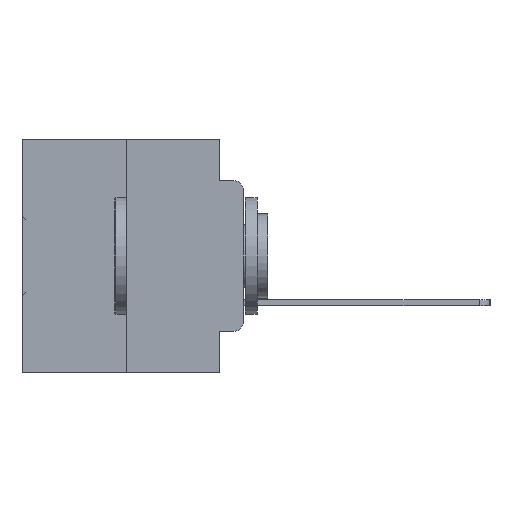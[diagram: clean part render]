
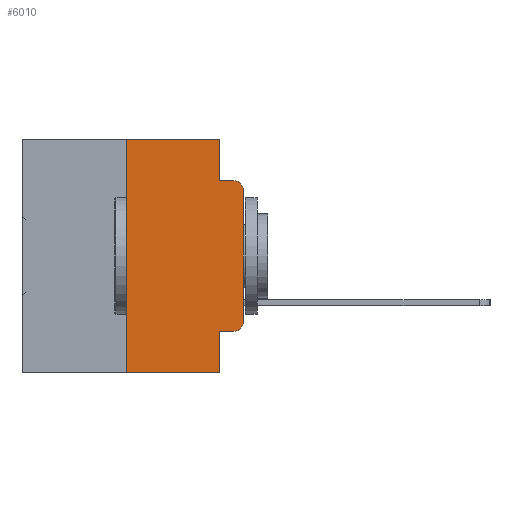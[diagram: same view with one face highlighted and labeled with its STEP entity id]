
A CAD part, left-side view. The second image highlights one B-rep face of the part: STEP entity #6010.
In plain terms, the highlighted planar face has unit normal (-1, 0, 0).
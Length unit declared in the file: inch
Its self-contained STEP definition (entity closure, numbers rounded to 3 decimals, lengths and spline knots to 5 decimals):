
#268 = CARTESIAN_POINT ( 'NONE',  ( 0., 0.25, 0. ) ) ;
#340 = VERTEX_POINT ( 'NONE', #10193 ) ;
#396 = DIRECTION ( 'NONE',  ( 0., 0., -1. ) ) ;
#1117 = LINE ( 'NONE', #17265, #7367 ) ;
#3021 = CARTESIAN_POINT ( 'NONE',  ( 0., 0.25, -0.5 ) ) ;
#3078 = CARTESIAN_POINT ( 'NONE',  ( 0., 0.02, -0.3915 ) ) ;
#4188 = EDGE_CURVE ( 'NONE', #33823, #26810, #32406, .T. ) ;
#4772 = DIRECTION ( 'NONE',  ( 0., -1., 0. ) ) ;
#4980 = VECTOR ( 'NONE', #13458, 39.37008 ) ;
#5019 = DIRECTION ( 'NONE',  ( 0., 0., -1. ) ) ;
#5294 = CARTESIAN_POINT ( 'NONE',  ( 0., 0.02, -0.0885 ) ) ;
#5438 = VERTEX_POINT ( 'NONE', #8675 ) ;
#5675 = CARTESIAN_POINT ( 'NONE',  ( 0., 0.051, 0. ) ) ;
#5756 = DIRECTION ( 'NONE',  ( 0., 0., -1. ) ) ;
#6002 = EDGE_CURVE ( 'NONE', #20664, #340, #11934, .T. ) ;
#6010 = ADVANCED_FACE ( 'NONE', ( #18909 ), #31740, .F. ) ;
#6214 = CARTESIAN_POINT ( 'NONE',  ( 0., 0.473, 0. ) ) ;
#6688 = VECTOR ( 'NONE', #8805, 39.37008 ) ;
#6819 = DIRECTION ( 'NONE',  ( 0., -1., 0. ) ) ;
#7367 = VECTOR ( 'NONE', #6819, 39.37008 ) ;
#7508 = LINE ( 'NONE', #6214, #6688 ) ;
#8301 = CIRCLE ( 'NONE', #22357, 0.02 ) ;
#8603 = VECTOR ( 'NONE', #4772, 39.37008 ) ;
#8675 = CARTESIAN_POINT ( 'NONE',  ( 0., 0.02, -0.4115 ) ) ;
#8805 = DIRECTION ( 'NONE',  ( 0., -1., 0. ) ) ;
#9456 = EDGE_CURVE ( 'NONE', #23991, #20001, #32070, .T. ) ;
#9887 = ORIENTED_EDGE ( 'NONE', *, *, #32769, .T. ) ;
#10193 = CARTESIAN_POINT ( 'NONE',  ( 0., 0.25, 0. ) ) ;
#10972 = CARTESIAN_POINT ( 'NONE',  ( 0., 0.051, -0.5 ) ) ;
#11659 = CARTESIAN_POINT ( 'NONE',  ( 0., 0.051, -0.4115 ) ) ;
#11934 = LINE ( 'NONE', #268, #4980 ) ;
#11980 = VERTEX_POINT ( 'NONE', #5294 ) ;
#12203 = CARTESIAN_POINT ( 'NONE',  ( 0., 0.02, -0.1085 ) ) ;
#12274 = LINE ( 'NONE', #32652, #19235 ) ;
#13046 = CARTESIAN_POINT ( 'NONE',  ( 0., 0.051, 0. ) ) ;
#13296 = AXIS2_PLACEMENT_3D ( 'NONE', #3078, #21322, #5756 ) ;
#13458 = DIRECTION ( 'NONE',  ( 0., 0., 1. ) ) ;
#14540 = DIRECTION ( 'NONE',  ( 0., -1., 0. ) ) ;
#14629 = EDGE_LOOP ( 'NONE', ( #31281, #31250, #31911, #31759, #32193, #31178, #17126, #23685, #9887, #17498 ) ) ;
#14752 = EDGE_CURVE ( 'NONE', #20001, #11980, #12274, .T. ) ;
#14838 = DIRECTION ( 'NONE',  ( 0., 0., -1. ) ) ;
#15705 = DIRECTION ( 'NONE',  ( 0., 0., -1. ) ) ;
#16242 = DIRECTION ( 'NONE',  ( 1., 0., 0. ) ) ;
#16294 = AXIS2_PLACEMENT_3D ( 'NONE', #23851, #16242, #396 ) ;
#17126 = ORIENTED_EDGE ( 'NONE', *, *, #17696, .T. ) ;
#17265 = CARTESIAN_POINT ( 'NONE',  ( 0., 0.051, -0.4115 ) ) ;
#17498 = ORIENTED_EDGE ( 'NONE', *, *, #31057, .T. ) ;
#17533 = DIRECTION ( 'NONE',  ( 0., 0., 1. ) ) ;
#17696 = EDGE_CURVE ( 'NONE', #20664, #26810, #30193, .T. ) ;
#18320 = VECTOR ( 'NONE', #15705, 39.37008 ) ;
#18909 = FACE_OUTER_BOUND ( 'NONE', #14629, .T. ) ;
#19235 = VECTOR ( 'NONE', #14540, 39.37008 ) ;
#19456 = VECTOR ( 'NONE', #5019, 39.37008 ) ;
#19981 = EDGE_CURVE ( 'NONE', #20700, #11980, #8301, .T. ) ;
#20001 = VERTEX_POINT ( 'NONE', #32971 ) ;
#20664 = VERTEX_POINT ( 'NONE', #3021 ) ;
#20700 = VERTEX_POINT ( 'NONE', #26618 ) ;
#21322 = DIRECTION ( 'NONE',  ( -1., 0., 0. ) ) ;
#21642 = EDGE_CURVE ( 'NONE', #32597, #20700, #23811, .T. ) ;
#22357 = AXIS2_PLACEMENT_3D ( 'NONE', #12203, #30387, #14838 ) ;
#22956 = CARTESIAN_POINT ( 'NONE',  ( 0., 0.473, -0.5 ) ) ;
#23685 = ORIENTED_EDGE ( 'NONE', *, *, #4188, .F. ) ;
#23811 = LINE ( 'NONE', #25253, #24636 ) ;
#23851 = CARTESIAN_POINT ( 'NONE',  ( 0., 0.473, 0. ) ) ;
#23991 = VERTEX_POINT ( 'NONE', #5675 ) ;
#24636 = VECTOR ( 'NONE', #17533, 39.37008 ) ;
#25253 = CARTESIAN_POINT ( 'NONE',  ( 0., 0., 0. ) ) ;
#26618 = CARTESIAN_POINT ( 'NONE',  ( 0., 0., -0.1085 ) ) ;
#26810 = VERTEX_POINT ( 'NONE', #10972 ) ;
#30193 = LINE ( 'NONE', #22956, #8603 ) ;
#30352 = CARTESIAN_POINT ( 'NONE',  ( 0., 0., -0.3915 ) ) ;
#30387 = DIRECTION ( 'NONE',  ( -1., 0., 0. ) ) ;
#31057 = EDGE_CURVE ( 'NONE', #5438, #32597, #31537, .T. ) ;
#31102 = CARTESIAN_POINT ( 'NONE',  ( 0., 0.051, 0. ) ) ;
#31168 = EDGE_CURVE ( 'NONE', #340, #23991, #7508, .T. ) ;
#31178 = ORIENTED_EDGE ( 'NONE', *, *, #6002, .F. ) ;
#31250 = ORIENTED_EDGE ( 'NONE', *, *, #19981, .T. ) ;
#31281 = ORIENTED_EDGE ( 'NONE', *, *, #21642, .T. ) ;
#31537 = CIRCLE ( 'NONE', #13296, 0.02 ) ;
#31740 = PLANE ( 'NONE',  #16294 ) ;
#31759 = ORIENTED_EDGE ( 'NONE', *, *, #9456, .F. ) ;
#31911 = ORIENTED_EDGE ( 'NONE', *, *, #14752, .F. ) ;
#32070 = LINE ( 'NONE', #13046, #18320 ) ;
#32193 = ORIENTED_EDGE ( 'NONE', *, *, #31168, .F. ) ;
#32406 = LINE ( 'NONE', #31102, #19456 ) ;
#32597 = VERTEX_POINT ( 'NONE', #30352 ) ;
#32652 = CARTESIAN_POINT ( 'NONE',  ( 0., 0.051, -0.0885 ) ) ;
#32769 = EDGE_CURVE ( 'NONE', #33823, #5438, #1117, .T. ) ;
#32971 = CARTESIAN_POINT ( 'NONE',  ( 0., 0.051, -0.0885 ) ) ;
#33823 = VERTEX_POINT ( 'NONE', #11659 ) ;
